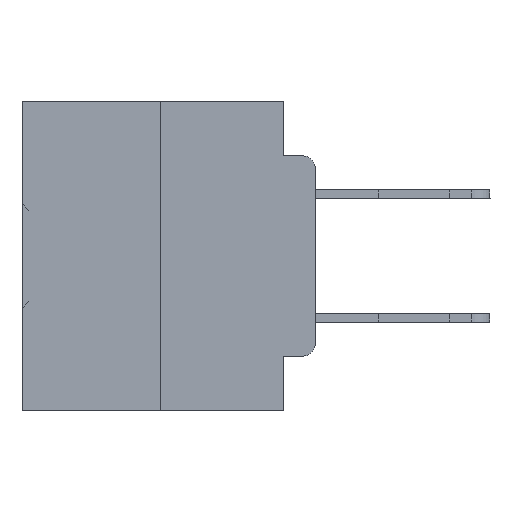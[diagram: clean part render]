
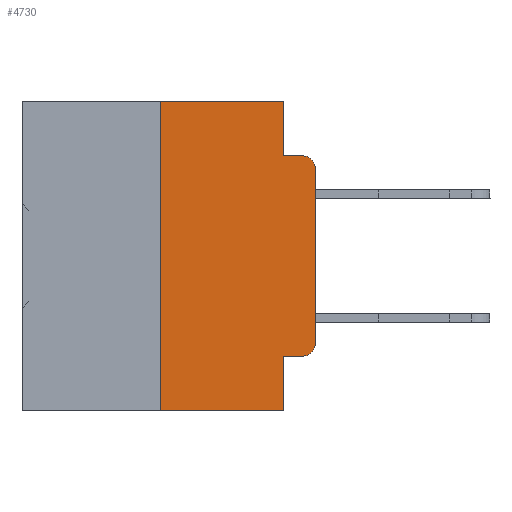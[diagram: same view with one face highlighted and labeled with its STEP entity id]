
A CAD part, left-side view. The second image highlights one B-rep face of the part: STEP entity #4730.
In plain terms, the highlighted planar face has unit normal (-1, 0, 0).
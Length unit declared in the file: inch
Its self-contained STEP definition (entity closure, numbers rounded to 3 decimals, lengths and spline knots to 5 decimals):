
#417 = ORIENTED_EDGE ( 'NONE', *, *, #18752, .F. ) ;
#1101 = CARTESIAN_POINT ( 'NONE',  ( 0., 0.051, -0.5 ) ) ;
#1951 = EDGE_CURVE ( 'NONE', #2421, #4589, #30408, .T. ) ;
#2321 = DIRECTION ( 'NONE',  ( 0., 0., -1. ) ) ;
#2421 = VERTEX_POINT ( 'NONE', #10020 ) ;
#2425 = LINE ( 'NONE', #36491, #17720 ) ;
#2934 = CARTESIAN_POINT ( 'NONE',  ( 0., 0., -0.1085 ) ) ;
#3265 = ORIENTED_EDGE ( 'NONE', *, *, #37178, .T. ) ;
#3306 = VERTEX_POINT ( 'NONE', #3308 ) ;
#3308 = CARTESIAN_POINT ( 'NONE',  ( 0., 0.051, -0.4115 ) ) ;
#4589 = VERTEX_POINT ( 'NONE', #34280 ) ;
#4668 = CARTESIAN_POINT ( 'NONE',  ( 0., 0.02, -0.3915 ) ) ;
#4730 = ADVANCED_FACE ( 'NONE', ( #7684 ), #6095, .F. ) ;
#6095 = PLANE ( 'NONE',  #6408 ) ;
#6206 = ORIENTED_EDGE ( 'NONE', *, *, #6562, .T. ) ;
#6408 = AXIS2_PLACEMENT_3D ( 'NONE', #6955, #7404, #13647 ) ;
#6562 = EDGE_CURVE ( 'NONE', #23168, #16194, #16561, .T. ) ;
#6791 = CARTESIAN_POINT ( 'NONE',  ( 0., 0.051, -0.0885 ) ) ;
#6955 = CARTESIAN_POINT ( 'NONE',  ( 0., 0.473, 0. ) ) ;
#7404 = DIRECTION ( 'NONE',  ( 1., 0., 0. ) ) ;
#7454 = DIRECTION ( 'NONE',  ( 0., -1., 0. ) ) ;
#7629 = LINE ( 'NONE', #22674, #22759 ) ;
#7684 = FACE_OUTER_BOUND ( 'NONE', #25826, .T. ) ;
#7779 = DIRECTION ( 'NONE',  ( 0., 0., -1. ) ) ;
#7796 = VERTEX_POINT ( 'NONE', #1101 ) ;
#8351 = LINE ( 'NONE', #26094, #31384 ) ;
#8604 = EDGE_CURVE ( 'NONE', #3306, #23168, #32591, .T. ) ;
#8652 = VECTOR ( 'NONE', #20074, 39.37008 ) ;
#10020 = CARTESIAN_POINT ( 'NONE',  ( 0., 0.25, 0. ) ) ;
#13647 = DIRECTION ( 'NONE',  ( 0., 0., -1. ) ) ;
#13994 = CARTESIAN_POINT ( 'NONE',  ( 0., 0.473, 0. ) ) ;
#14269 = VECTOR ( 'NONE', #24585, 39.37008 ) ;
#14586 = VECTOR ( 'NONE', #33465, 39.37008 ) ;
#14750 = EDGE_CURVE ( 'NONE', #3306, #7796, #19093, .T. ) ;
#15414 = CARTESIAN_POINT ( 'NONE',  ( 0., 0.051, 0. ) ) ;
#15788 = VERTEX_POINT ( 'NONE', #26209 ) ;
#16194 = VERTEX_POINT ( 'NONE', #27967 ) ;
#16561 = CIRCLE ( 'NONE', #16893, 0.02 ) ;
#16766 = EDGE_CURVE ( 'NONE', #15788, #2421, #24442, .T. ) ;
#16893 = AXIS2_PLACEMENT_3D ( 'NONE', #4668, #25853, #7779 ) ;
#17048 = CARTESIAN_POINT ( 'NONE',  ( 0., 0.051, -0.4115 ) ) ;
#17720 = VECTOR ( 'NONE', #21725, 39.37008 ) ;
#18752 = EDGE_CURVE ( 'NONE', #4589, #25370, #2425, .T. ) ;
#19093 = LINE ( 'NONE', #15414, #14269 ) ;
#20074 = DIRECTION ( 'NONE',  ( 0., -1., 0. ) ) ;
#20572 = DIRECTION ( 'NONE',  ( -1., 0., 0. ) ) ;
#21614 = VERTEX_POINT ( 'NONE', #24693 ) ;
#21725 = DIRECTION ( 'NONE',  ( 0., 0., -1. ) ) ;
#21822 = ORIENTED_EDGE ( 'NONE', *, *, #28806, .T. ) ;
#22674 = CARTESIAN_POINT ( 'NONE',  ( 0., 0., 0. ) ) ;
#22759 = VECTOR ( 'NONE', #25668, 39.37008 ) ;
#23168 = VERTEX_POINT ( 'NONE', #37752 ) ;
#23946 = AXIS2_PLACEMENT_3D ( 'NONE', #38301, #20572, #2321 ) ;
#24442 = LINE ( 'NONE', #33584, #14586 ) ;
#24585 = DIRECTION ( 'NONE',  ( 0., 0., -1. ) ) ;
#24636 = ORIENTED_EDGE ( 'NONE', *, *, #1951, .F. ) ;
#24693 = CARTESIAN_POINT ( 'NONE',  ( 0., 0.02, -0.0885 ) ) ;
#25370 = VERTEX_POINT ( 'NONE', #6791 ) ;
#25668 = DIRECTION ( 'NONE',  ( 0., 0., 1. ) ) ;
#25826 = EDGE_LOOP ( 'NONE', ( #27872, #21822, #37570, #417, #24636, #32518, #3265, #27423, #29322, #6206 ) ) ;
#25853 = DIRECTION ( 'NONE',  ( -1., 0., 0. ) ) ;
#26094 = CARTESIAN_POINT ( 'NONE',  ( 0., 0.051, -0.0885 ) ) ;
#26209 = CARTESIAN_POINT ( 'NONE',  ( 0., 0.25, -0.5 ) ) ;
#26805 = EDGE_CURVE ( 'NONE', #25370, #21614, #8351, .T. ) ;
#27017 = CIRCLE ( 'NONE', #23946, 0.02 ) ;
#27423 = ORIENTED_EDGE ( 'NONE', *, *, #14750, .F. ) ;
#27872 = ORIENTED_EDGE ( 'NONE', *, *, #34700, .T. ) ;
#27967 = CARTESIAN_POINT ( 'NONE',  ( 0., 0., -0.3915 ) ) ;
#28806 = EDGE_CURVE ( 'NONE', #32601, #21614, #27017, .T. ) ;
#29075 = DIRECTION ( 'NONE',  ( 0., -1., 0. ) ) ;
#29322 = ORIENTED_EDGE ( 'NONE', *, *, #8604, .T. ) ;
#30408 = LINE ( 'NONE', #13994, #36366 ) ;
#31384 = VECTOR ( 'NONE', #29075, 39.37008 ) ;
#32518 = ORIENTED_EDGE ( 'NONE', *, *, #16766, .F. ) ;
#32591 = LINE ( 'NONE', #17048, #8652 ) ;
#32601 = VERTEX_POINT ( 'NONE', #2934 ) ;
#33124 = CARTESIAN_POINT ( 'NONE',  ( 0., 0.473, -0.5 ) ) ;
#33465 = DIRECTION ( 'NONE',  ( 0., 0., 1. ) ) ;
#33584 = CARTESIAN_POINT ( 'NONE',  ( 0., 0.25, 0. ) ) ;
#34280 = CARTESIAN_POINT ( 'NONE',  ( 0., 0.051, 0. ) ) ;
#34700 = EDGE_CURVE ( 'NONE', #16194, #32601, #7629, .T. ) ;
#36088 = DIRECTION ( 'NONE',  ( 0., -1., 0. ) ) ;
#36366 = VECTOR ( 'NONE', #7454, 39.37008 ) ;
#36491 = CARTESIAN_POINT ( 'NONE',  ( 0., 0.051, 0. ) ) ;
#37178 = EDGE_CURVE ( 'NONE', #15788, #7796, #38697, .T. ) ;
#37570 = ORIENTED_EDGE ( 'NONE', *, *, #26805, .F. ) ;
#37752 = CARTESIAN_POINT ( 'NONE',  ( 0., 0.02, -0.4115 ) ) ;
#37810 = VECTOR ( 'NONE', #36088, 39.37008 ) ;
#38301 = CARTESIAN_POINT ( 'NONE',  ( 0., 0.02, -0.1085 ) ) ;
#38697 = LINE ( 'NONE', #33124, #37810 ) ;
